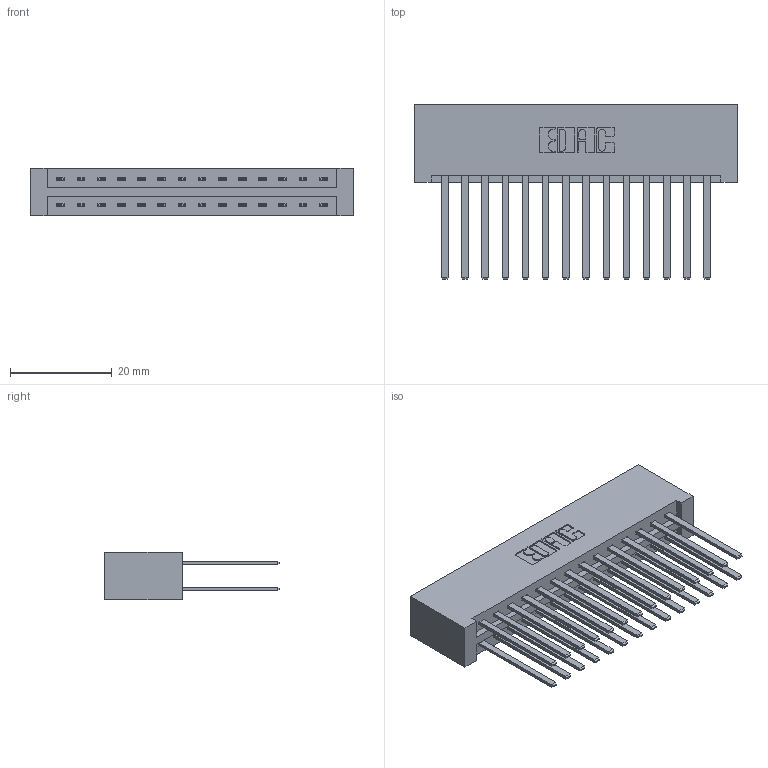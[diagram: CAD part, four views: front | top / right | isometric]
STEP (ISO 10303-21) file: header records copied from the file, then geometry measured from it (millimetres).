
FILE_DESCRIPTION (( 'STEP AP203' ), '1' );
FILE_NAME ('337-028-544-201.STEP', '2019-10-08T17:08:50', ( '' ), ( '' ), 'SwSTEP 2.0', 'SolidWorks 2016', '' );
FILE_SCHEMA (( 'CONFIG_CONTROL_DESIGN' ));
Length unit declared in the file: inch
Products named in the file (3): 337-028-544-201; 345-292-001_345-293-144; 337 Part_No Mounting Lugs
Assembly tree (29 placements, depth 2):
  337-028-544-201
    337 Part_No Mounting Lugs
    345-292-001_345-293-144  x28
Bounding box: 63.35 x 34.3 x 9.4 mm (x, y, z)
Volume: 7456.6 mm3; surface area: 9496 mm2
Topology: 29 solids, 29 shells, 1450 faces, 4291 edges, 2822 vertices
Faces by surface type: plane 1018, cylinder 432
Entity records: 14015 total; most frequent: CARTESIAN_POINT 2382, ORIENTED_EDGE 2318, DIRECTION 2067, EDGE_CURVE 1159, LINE 1043, VECTOR 1043, VERTEX_POINT 770, AXIS2_PLACEMENT_3D 512
